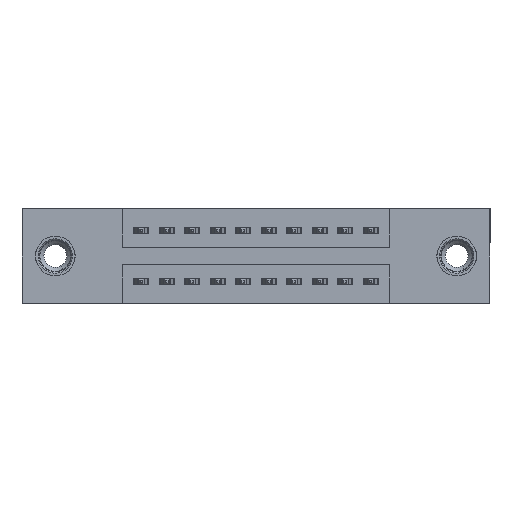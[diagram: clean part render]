
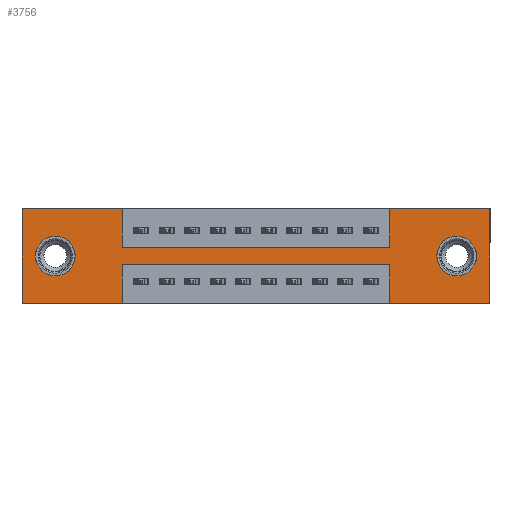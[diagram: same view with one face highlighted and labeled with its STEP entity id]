
A CAD part, front view. The second image highlights one B-rep face of the part: STEP entity #3756.
In plain terms, the highlighted planar face has unit normal (0, -1, 0).
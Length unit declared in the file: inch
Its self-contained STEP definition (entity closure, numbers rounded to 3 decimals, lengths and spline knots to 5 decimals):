
#248 = VERTEX_POINT ( 'NONE', #3324 ) ;
#288 = AXIS2_PLACEMENT_3D ( 'NONE', #4059, #11793, #5189 ) ;
#408 = VERTEX_POINT ( 'NONE', #6989 ) ;
#690 = ORIENTED_EDGE ( 'NONE', *, *, #6130, .F. ) ;
#720 = VERTEX_POINT ( 'NONE', #12185 ) ;
#800 = PLANE ( 'NONE',  #2929 ) ;
#810 = LINE ( 'NONE', #5159, #12269 ) ;
#973 = EDGE_CURVE ( 'NONE', #720, #8945, #8385, .T. ) ;
#1045 = CARTESIAN_POINT ( 'NONE',  ( 1.4425, 0., 0. ) ) ;
#1058 = EDGE_LOOP ( 'NONE', ( #13666, #8225 ) ) ;
#1332 = LINE ( 'NONE', #5025, #3598 ) ;
#1335 = FACE_BOUND ( 'NONE', #6361, .T. ) ;
#1399 = ORIENTED_EDGE ( 'NONE', *, *, #973, .F. ) ;
#1456 = DIRECTION ( 'NONE',  ( 0., 0., -1. ) ) ;
#1508 = DIRECTION ( 'NONE',  ( 0., 1., 0. ) ) ;
#1629 = VECTOR ( 'NONE', #7619, 39.37008 ) ;
#1668 = VECTOR ( 'NONE', #2032, 39.37008 ) ;
#1755 = ORIENTED_EDGE ( 'NONE', *, *, #12280, .F. ) ;
#1922 = ORIENTED_EDGE ( 'NONE', *, *, #12557, .T. ) ;
#1941 = DIRECTION ( 'NONE',  ( 0., 0., -1. ) ) ;
#2032 = DIRECTION ( 'NONE',  ( 0., 0., -1. ) ) ;
#2633 = DIRECTION ( 'NONE',  ( 1., 0., 0. ) ) ;
#2635 = ORIENTED_EDGE ( 'NONE', *, *, #11410, .F. ) ;
#2728 = VERTEX_POINT ( 'NONE', #4418 ) ;
#2803 = EDGE_LOOP ( 'NONE', ( #2635, #8569, #14202, #5929, #6274, #12158, #690, #12487, #1399, #7350, #13173, #1755 ) ) ;
#2907 = LINE ( 'NONE', #7059, #8498 ) ;
#2929 = AXIS2_PLACEMENT_3D ( 'NONE', #11869, #8629, #1941 ) ;
#3023 = EDGE_CURVE ( 'NONE', #248, #11513, #5222, .T. ) ;
#3115 = DIRECTION ( 'NONE',  ( 0., 1., 0. ) ) ;
#3135 = VECTOR ( 'NONE', #1456, 39.37008 ) ;
#3148 = CARTESIAN_POINT ( 'NONE',  ( 0.13, 0., -0.107 ) ) ;
#3282 = CARTESIAN_POINT ( 'NONE',  ( 1.4425, 0., -0.37 ) ) ;
#3324 = CARTESIAN_POINT ( 'NONE',  ( 1.835, 0., -0.37 ) ) ;
#3598 = VECTOR ( 'NONE', #13820, 39.37008 ) ;
#3657 = LINE ( 'NONE', #7071, #9279 ) ;
#3713 = CIRCLE ( 'NONE', #11805, 0.078 ) ;
#3756 = ADVANCED_FACE ( 'NONE', ( #1335, #4673, #4331 ), #800, .T. ) ;
#3794 = DIRECTION ( 'NONE',  ( -1., 0., 0. ) ) ;
#4059 = CARTESIAN_POINT ( 'NONE',  ( 1.705, 0., -0.185 ) ) ;
#4275 = VECTOR ( 'NONE', #9336, 39.37008 ) ;
#4310 = CARTESIAN_POINT ( 'NONE',  ( 0.3925, 0., 0. ) ) ;
#4331 = FACE_OUTER_BOUND ( 'NONE', #2803, .T. ) ;
#4418 = CARTESIAN_POINT ( 'NONE',  ( 1.4425, 0., -0.15 ) ) ;
#4533 = LINE ( 'NONE', #13677, #9417 ) ;
#4549 = ORIENTED_EDGE ( 'NONE', *, *, #5056, .T. ) ;
#4600 = EDGE_CURVE ( 'NONE', #5809, #12116, #1332, .T. ) ;
#4673 = FACE_BOUND ( 'NONE', #1058, .T. ) ;
#4842 = CARTESIAN_POINT ( 'NONE',  ( 0., 0., -0.37 ) ) ;
#4879 = DIRECTION ( 'NONE',  ( 0., 0., 1. ) ) ;
#5025 = CARTESIAN_POINT ( 'NONE',  ( 0., 0., 0. ) ) ;
#5056 = EDGE_CURVE ( 'NONE', #13184, #12573, #10527, .T. ) ;
#5159 = CARTESIAN_POINT ( 'NONE',  ( 0.3925, 0., -0.15 ) ) ;
#5189 = DIRECTION ( 'NONE',  ( 0., 0., -1. ) ) ;
#5222 = LINE ( 'NONE', #8312, #13636 ) ;
#5670 = CARTESIAN_POINT ( 'NONE',  ( 1.835, 0., 0. ) ) ;
#5755 = AXIS2_PLACEMENT_3D ( 'NONE', #6288, #13976, #7435 ) ;
#5801 = VECTOR ( 'NONE', #11019, 39.37008 ) ;
#5809 = VERTEX_POINT ( 'NONE', #8308 ) ;
#5929 = ORIENTED_EDGE ( 'NONE', *, *, #3023, .F. ) ;
#6021 = VERTEX_POINT ( 'NONE', #11916 ) ;
#6047 = EDGE_CURVE ( 'NONE', #408, #7788, #9832, .T. ) ;
#6130 = EDGE_CURVE ( 'NONE', #2728, #5809, #14235, .T. ) ;
#6274 = ORIENTED_EDGE ( 'NONE', *, *, #7714, .F. ) ;
#6288 = CARTESIAN_POINT ( 'NONE',  ( 0.13, 0., -0.185 ) ) ;
#6306 = DIRECTION ( 'NONE',  ( 0., 0., 1. ) ) ;
#6361 = EDGE_LOOP ( 'NONE', ( #4549, #1922 ) ) ;
#6614 = EDGE_CURVE ( 'NONE', #11513, #408, #10990, .T. ) ;
#6737 = VERTEX_POINT ( 'NONE', #3148 ) ;
#6779 = CARTESIAN_POINT ( 'NONE',  ( 0.13, 0., -0.263 ) ) ;
#6961 = VERTEX_POINT ( 'NONE', #7990 ) ;
#6989 = CARTESIAN_POINT ( 'NONE',  ( 1.4425, 0., -0.22 ) ) ;
#7059 = CARTESIAN_POINT ( 'NONE',  ( 0., 0., 0. ) ) ;
#7071 = CARTESIAN_POINT ( 'NONE',  ( 1.835, 0., 0. ) ) ;
#7145 = CIRCLE ( 'NONE', #11404, 0.078 ) ;
#7175 = CARTESIAN_POINT ( 'NONE',  ( 0.3925, 0., -0.22 ) ) ;
#7228 = LINE ( 'NONE', #4842, #4275 ) ;
#7257 = LINE ( 'NONE', #8719, #1668 ) ;
#7322 = CARTESIAN_POINT ( 'NONE',  ( 0.3925, 0., -0.15 ) ) ;
#7342 = CARTESIAN_POINT ( 'NONE',  ( 0., 0., -0.37 ) ) ;
#7350 = ORIENTED_EDGE ( 'NONE', *, *, #11103, .F. ) ;
#7435 = DIRECTION ( 'NONE',  ( 0., 0., 1. ) ) ;
#7609 = VERTEX_POINT ( 'NONE', #6779 ) ;
#7619 = DIRECTION ( 'NONE',  ( -1., 0., 0. ) ) ;
#7714 = EDGE_CURVE ( 'NONE', #12116, #248, #3657, .T. ) ;
#7788 = VERTEX_POINT ( 'NONE', #7175 ) ;
#7990 = CARTESIAN_POINT ( 'NONE',  ( 0.3925, 0., -0.37 ) ) ;
#8216 = CARTESIAN_POINT ( 'NONE',  ( 0.13, 0., -0.185 ) ) ;
#8217 = DIRECTION ( 'NONE',  ( 0., 0., -1. ) ) ;
#8225 = ORIENTED_EDGE ( 'NONE', *, *, #8782, .T. ) ;
#8281 = VERTEX_POINT ( 'NONE', #7342 ) ;
#8308 = CARTESIAN_POINT ( 'NONE',  ( 1.4425, 0., 0. ) ) ;
#8312 = CARTESIAN_POINT ( 'NONE',  ( 0., 0., -0.37 ) ) ;
#8330 = EDGE_CURVE ( 'NONE', #6737, #7609, #8566, .T. ) ;
#8385 = LINE ( 'NONE', #4310, #3135 ) ;
#8429 = VECTOR ( 'NONE', #6306, 39.37008 ) ;
#8498 = VECTOR ( 'NONE', #2633, 39.37008 ) ;
#8566 = CIRCLE ( 'NONE', #5755, 0.078 ) ;
#8569 = ORIENTED_EDGE ( 'NONE', *, *, #6047, .F. ) ;
#8629 = DIRECTION ( 'NONE',  ( 0., -1., 0. ) ) ;
#8675 = CARTESIAN_POINT ( 'NONE',  ( 1.705, 0., -0.107 ) ) ;
#8719 = CARTESIAN_POINT ( 'NONE',  ( 0.3925, 0., -0.37 ) ) ;
#8782 = EDGE_CURVE ( 'NONE', #7609, #6737, #7145, .T. ) ;
#8820 = EDGE_CURVE ( 'NONE', #8281, #6021, #4533, .T. ) ;
#8945 = VERTEX_POINT ( 'NONE', #7322 ) ;
#9279 = VECTOR ( 'NONE', #8217, 39.37008 ) ;
#9330 = DIRECTION ( 'NONE',  ( 0., 0., 1. ) ) ;
#9336 = DIRECTION ( 'NONE',  ( -1., 0., 0. ) ) ;
#9417 = VECTOR ( 'NONE', #4879, 39.37008 ) ;
#9694 = EDGE_CURVE ( 'NONE', #8945, #2728, #810, .T. ) ;
#9805 = CARTESIAN_POINT ( 'NONE',  ( 1.705, 0., -0.185 ) ) ;
#9832 = LINE ( 'NONE', #14154, #1629 ) ;
#10527 = CIRCLE ( 'NONE', #288, 0.078 ) ;
#10882 = DIRECTION ( 'NONE',  ( 0., 0., -1. ) ) ;
#10990 = LINE ( 'NONE', #12905, #8429 ) ;
#11019 = DIRECTION ( 'NONE',  ( 0., 0., 1. ) ) ;
#11103 = EDGE_CURVE ( 'NONE', #6021, #720, #2907, .T. ) ;
#11404 = AXIS2_PLACEMENT_3D ( 'NONE', #8216, #1508, #9330 ) ;
#11410 = EDGE_CURVE ( 'NONE', #7788, #6961, #7257, .T. ) ;
#11513 = VERTEX_POINT ( 'NONE', #3282 ) ;
#11793 = DIRECTION ( 'NONE',  ( 0., 1., 0. ) ) ;
#11805 = AXIS2_PLACEMENT_3D ( 'NONE', #9805, #3115, #10882 ) ;
#11869 = CARTESIAN_POINT ( 'NONE',  ( 0., 0., -0.37 ) ) ;
#11916 = CARTESIAN_POINT ( 'NONE',  ( 0., 0., 0. ) ) ;
#12116 = VERTEX_POINT ( 'NONE', #5670 ) ;
#12158 = ORIENTED_EDGE ( 'NONE', *, *, #4600, .F. ) ;
#12185 = CARTESIAN_POINT ( 'NONE',  ( 0.3925, 0., 0. ) ) ;
#12269 = VECTOR ( 'NONE', #13941, 39.37008 ) ;
#12280 = EDGE_CURVE ( 'NONE', #6961, #8281, #7228, .T. ) ;
#12487 = ORIENTED_EDGE ( 'NONE', *, *, #9694, .F. ) ;
#12557 = EDGE_CURVE ( 'NONE', #12573, #13184, #3713, .T. ) ;
#12573 = VERTEX_POINT ( 'NONE', #14155 ) ;
#12905 = CARTESIAN_POINT ( 'NONE',  ( 1.4425, 0., -0.37 ) ) ;
#13173 = ORIENTED_EDGE ( 'NONE', *, *, #8820, .F. ) ;
#13184 = VERTEX_POINT ( 'NONE', #8675 ) ;
#13636 = VECTOR ( 'NONE', #3794, 39.37008 ) ;
#13666 = ORIENTED_EDGE ( 'NONE', *, *, #8330, .T. ) ;
#13677 = CARTESIAN_POINT ( 'NONE',  ( 0., 0., 0. ) ) ;
#13820 = DIRECTION ( 'NONE',  ( 1., 0., 0. ) ) ;
#13941 = DIRECTION ( 'NONE',  ( 1., 0., 0. ) ) ;
#13976 = DIRECTION ( 'NONE',  ( 0., 1., 0. ) ) ;
#14154 = CARTESIAN_POINT ( 'NONE',  ( 0.3925, 0., -0.22 ) ) ;
#14155 = CARTESIAN_POINT ( 'NONE',  ( 1.705, 0., -0.263 ) ) ;
#14202 = ORIENTED_EDGE ( 'NONE', *, *, #6614, .F. ) ;
#14235 = LINE ( 'NONE', #1045, #5801 ) ;
